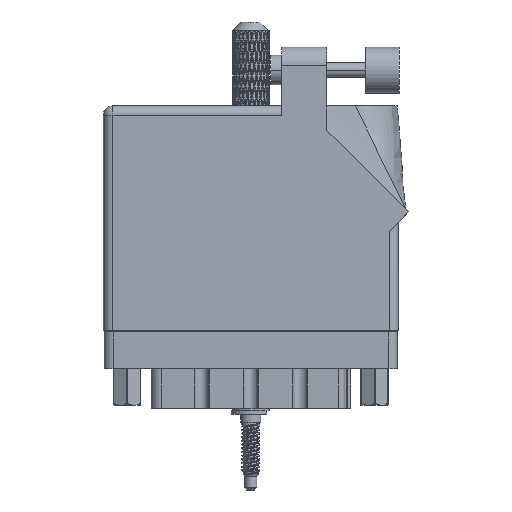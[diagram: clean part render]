
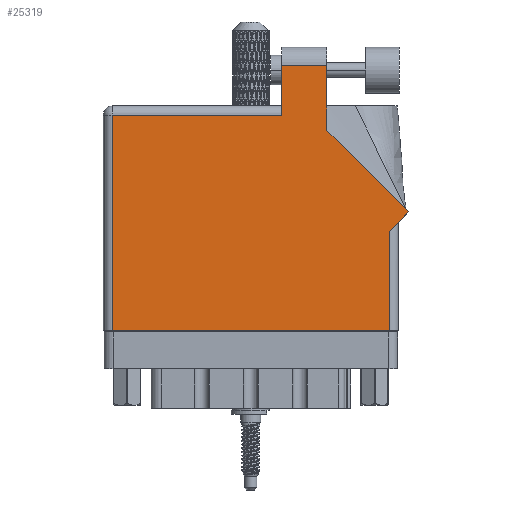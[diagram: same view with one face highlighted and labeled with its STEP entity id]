
A CAD part, front view. The second image highlights one B-rep face of the part: STEP entity #25319.
In plain terms, the highlighted face is planar.
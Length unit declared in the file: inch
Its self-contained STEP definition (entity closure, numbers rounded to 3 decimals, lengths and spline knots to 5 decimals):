
#3017 = ORIENTED_EDGE ( 'NONE', *, *, #21253, .T. ) ;
#3774 = CARTESIAN_POINT ( 'NONE',  ( 1.948, 0.737, 0. ) ) ;
#7624 = CARTESIAN_POINT ( 'NONE',  ( 1.217, 1.805, 0. ) ) ;
#7867 = CARTESIAN_POINT ( 'NONE',  ( 1.524, 1.805, 0. ) ) ;
#10757 = AXIS2_PLACEMENT_3D ( 'NONE', #113464, #15902, #69760 ) ;
#12050 = VERTEX_POINT ( 'NONE', #36243 ) ;
#12139 = CARTESIAN_POINT ( 'NONE',  ( 1.948, 0., 0. ) ) ;
#12705 = ORIENTED_EDGE ( 'NONE', *, *, #108665, .T. ) ;
#13800 = CARTESIAN_POINT ( 'NONE',  ( 0., 1.468, 0. ) ) ;
#15466 = VERTEX_POINT ( 'NONE', #12139 ) ;
#15902 = DIRECTION ( 'NONE',  ( 0., 0., -1. ) ) ;
#17796 = ORIENTED_EDGE ( 'NONE', *, *, #65081, .T. ) ;
#17801 = VERTEX_POINT ( 'NONE', #54839 ) ;
#18232 = VECTOR ( 'NONE', #81103, 39.37008 ) ;
#21125 = EDGE_LOOP ( 'NONE', ( #98705, #43819, #12705, #87933, #81923, #22987, #17796, #3017, #23473 ) ) ;
#21253 = EDGE_CURVE ( 'NONE', #17801, #55917, #65710, .T. ) ;
#21494 = LINE ( 'NONE', #3774, #42527 ) ;
#21650 = DIRECTION ( 'NONE',  ( 0., -1., 0. ) ) ;
#22752 = DIRECTION ( 'NONE',  ( -1., 0., 0. ) ) ;
#22933 = DIRECTION ( 'NONE',  ( -0.707, 0.707, 0. ) ) ;
#22987 = ORIENTED_EDGE ( 'NONE', *, *, #81446, .T. ) ;
#23473 = ORIENTED_EDGE ( 'NONE', *, *, #89794, .T. ) ;
#23771 = LINE ( 'NONE', #115726, #40642 ) ;
#25319 = ADVANCED_FACE ( 'NONE', ( #95883 ), #113848, .F. ) ;
#26287 = VECTOR ( 'NONE', #62727, 39.37008 ) ;
#28705 = CARTESIAN_POINT ( 'NONE',  ( 2.01, 0.737, 0. ) ) ;
#29117 = LINE ( 'NONE', #13800, #36132 ) ;
#33333 = LINE ( 'NONE', #103013, #54346 ) ;
#36132 = VECTOR ( 'NONE', #22752, 39.37008 ) ;
#36243 = CARTESIAN_POINT ( 'NONE',  ( 0.062, 0., 0. ) ) ;
#38035 = CARTESIAN_POINT ( 'NONE',  ( 1.524, 1.36442, 0. ) ) ;
#39202 = LINE ( 'NONE', #75300, #108927 ) ;
#39874 = EDGE_CURVE ( 'NONE', #50405, #110325, #29117, .T. ) ;
#40642 = VECTOR ( 'NONE', #107522, 39.37008 ) ;
#42527 = VECTOR ( 'NONE', #57220, 39.37008 ) ;
#43658 = VECTOR ( 'NONE', #21650, 39.37008 ) ;
#43819 = ORIENTED_EDGE ( 'NONE', *, *, #53626, .T. ) ;
#50405 = VERTEX_POINT ( 'NONE', #97391 ) ;
#52633 = CARTESIAN_POINT ( 'NONE',  ( 1.524, 1.36442, 0. ) ) ;
#53626 = EDGE_CURVE ( 'NONE', #82606, #104398, #65371, .T. ) ;
#54228 = VECTOR ( 'NONE', #61116, 39.37008 ) ;
#54346 = VECTOR ( 'NONE', #22933, 39.37008 ) ;
#54839 = CARTESIAN_POINT ( 'NONE',  ( 1.948, 0.675, 0. ) ) ;
#55917 = VERTEX_POINT ( 'NONE', #84259 ) ;
#57220 = DIRECTION ( 'NONE',  ( 0., 1., 0. ) ) ;
#61116 = DIRECTION ( 'NONE',  ( -1., 0., 0. ) ) ;
#62727 = DIRECTION ( 'NONE',  ( 0., 1., 0. ) ) ;
#65081 = EDGE_CURVE ( 'NONE', #15466, #17801, #21494, .T. ) ;
#65371 = LINE ( 'NONE', #7624, #54228 ) ;
#65710 = LINE ( 'NONE', #28705, #18232 ) ;
#67044 = DIRECTION ( 'NONE',  ( 1., 0., 0. ) ) ;
#69250 = EDGE_CURVE ( 'NONE', #110325, #12050, #23771, .T. ) ;
#69760 = DIRECTION ( 'NONE',  ( -1., 0., 0. ) ) ;
#75300 = CARTESIAN_POINT ( 'NONE',  ( 0., 0., 0. ) ) ;
#81103 = DIRECTION ( 'NONE',  ( 0.707, 0.707, 0. ) ) ;
#81446 = EDGE_CURVE ( 'NONE', #12050, #15466, #39202, .T. ) ;
#81923 = ORIENTED_EDGE ( 'NONE', *, *, #69250, .T. ) ;
#82606 = VERTEX_POINT ( 'NONE', #7867 ) ;
#82634 = CARTESIAN_POINT ( 'NONE',  ( 1.217, 1.53, 0. ) ) ;
#83132 = EDGE_CURVE ( 'NONE', #95301, #82606, #110060, .T. ) ;
#84259 = CARTESIAN_POINT ( 'NONE',  ( 2.08071, 0.80771, 0. ) ) ;
#87933 = ORIENTED_EDGE ( 'NONE', *, *, #39874, .T. ) ;
#88174 = CARTESIAN_POINT ( 'NONE',  ( 0.062, 1.468, 0. ) ) ;
#88349 = LINE ( 'NONE', #82634, #43658 ) ;
#89794 = EDGE_CURVE ( 'NONE', #55917, #95301, #33333, .T. ) ;
#95301 = VERTEX_POINT ( 'NONE', #38035 ) ;
#95883 = FACE_OUTER_BOUND ( 'NONE', #21125, .T. ) ;
#97391 = CARTESIAN_POINT ( 'NONE',  ( 1.217, 1.468, 0. ) ) ;
#98705 = ORIENTED_EDGE ( 'NONE', *, *, #83132, .T. ) ;
#103013 = CARTESIAN_POINT ( 'NONE',  ( 2.08071, 0.80771, 0. ) ) ;
#104398 = VERTEX_POINT ( 'NONE', #114546 ) ;
#107522 = DIRECTION ( 'NONE',  ( 0., -1., 0. ) ) ;
#108665 = EDGE_CURVE ( 'NONE', #104398, #50405, #88349, .T. ) ;
#108927 = VECTOR ( 'NONE', #67044, 39.37008 ) ;
#110060 = LINE ( 'NONE', #52633, #26287 ) ;
#110325 = VERTEX_POINT ( 'NONE', #88174 ) ;
#113464 = CARTESIAN_POINT ( 'NONE',  ( 0., 1.53, 0. ) ) ;
#113848 = PLANE ( 'NONE',  #10757 ) ;
#114546 = CARTESIAN_POINT ( 'NONE',  ( 1.217, 1.805, 0. ) ) ;
#115726 = CARTESIAN_POINT ( 'NONE',  ( 0.062, 0., 0. ) ) ;
